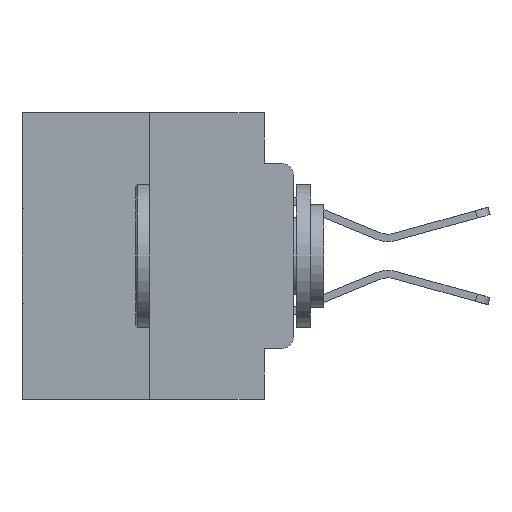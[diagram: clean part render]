
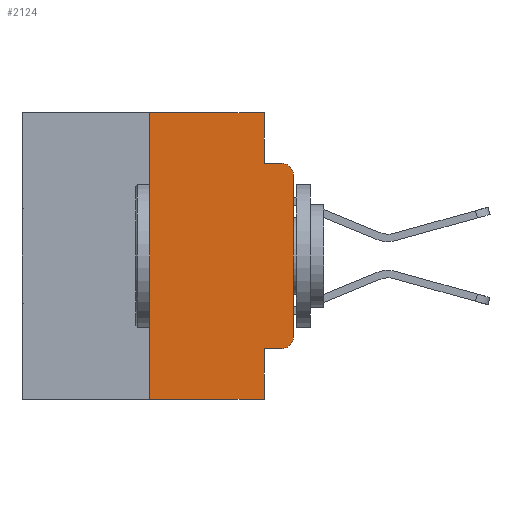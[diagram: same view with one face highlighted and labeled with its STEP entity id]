
A CAD part, left-side view. The second image highlights one B-rep face of the part: STEP entity #2124.
In plain terms, the highlighted planar face has unit normal (-1, 0, 0).
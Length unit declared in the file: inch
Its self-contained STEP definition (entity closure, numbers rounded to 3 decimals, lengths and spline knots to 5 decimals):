
#1100 = CARTESIAN_POINT ( 'NONE',  ( 0., 0.02, -0.4115 ) ) ;
#1102 = CARTESIAN_POINT ( 'NONE',  ( 0., 0., -0.3915 ) ) ;
#1301 = VERTEX_POINT ( 'NONE', #28978 ) ;
#1365 = DIRECTION ( 'NONE',  ( 0., 0., -1. ) ) ;
#1378 = EDGE_CURVE ( 'NONE', #5796, #15668, #2457, .T. ) ;
#1748 = CARTESIAN_POINT ( 'NONE',  ( 0., 0.25, 0. ) ) ;
#1887 = CARTESIAN_POINT ( 'NONE',  ( 0., 0.051, -0.0885 ) ) ;
#1997 = DIRECTION ( 'NONE',  ( -1., 0., 0. ) ) ;
#2112 = ORIENTED_EDGE ( 'NONE', *, *, #6102, .T. ) ;
#2124 = ADVANCED_FACE ( 'NONE', ( #12928 ), #16229, .F. ) ;
#2457 = LINE ( 'NONE', #1887, #20189 ) ;
#2640 = DIRECTION ( 'NONE',  ( 0., -1., 0. ) ) ;
#2888 = CARTESIAN_POINT ( 'NONE',  ( 0., 0.051, -0.0885 ) ) ;
#3114 = LINE ( 'NONE', #1748, #26795 ) ;
#3273 = VECTOR ( 'NONE', #23476, 39.37008 ) ;
#3896 = CARTESIAN_POINT ( 'NONE',  ( 0., 0.051, -0.4115 ) ) ;
#4103 = VECTOR ( 'NONE', #1365, 39.37008 ) ;
#4521 = EDGE_CURVE ( 'NONE', #17932, #15668, #16474, .T. ) ;
#4847 = LINE ( 'NONE', #28804, #4103 ) ;
#5796 = VERTEX_POINT ( 'NONE', #2888 ) ;
#6102 = EDGE_CURVE ( 'NONE', #15426, #17932, #23498, .T. ) ;
#6878 = ORIENTED_EDGE ( 'NONE', *, *, #26819, .T. ) ;
#6981 = VECTOR ( 'NONE', #29676, 39.37008 ) ;
#7036 = CARTESIAN_POINT ( 'NONE',  ( 0., 0.473, 0. ) ) ;
#7969 = AXIS2_PLACEMENT_3D ( 'NONE', #15907, #1997, #18211 ) ;
#8271 = EDGE_CURVE ( 'NONE', #11096, #24901, #26843, .T. ) ;
#9489 = CARTESIAN_POINT ( 'NONE',  ( 0., 0.473, 0. ) ) ;
#9795 = EDGE_CURVE ( 'NONE', #24345, #18157, #3114, .T. ) ;
#10985 = DIRECTION ( 'NONE',  ( 0., -1., 0. ) ) ;
#11096 = VERTEX_POINT ( 'NONE', #3896 ) ;
#11794 = DIRECTION ( 'NONE',  ( 0., 0., -1. ) ) ;
#12287 = ORIENTED_EDGE ( 'NONE', *, *, #28628, .T. ) ;
#12374 = CARTESIAN_POINT ( 'NONE',  ( 0., 0.25, 0. ) ) ;
#12656 = DIRECTION ( 'NONE',  ( -1., 0., 0. ) ) ;
#12928 = FACE_OUTER_BOUND ( 'NONE', #15878, .T. ) ;
#15426 = VERTEX_POINT ( 'NONE', #1102 ) ;
#15502 = ORIENTED_EDGE ( 'NONE', *, *, #4521, .T. ) ;
#15606 = LINE ( 'NONE', #21165, #3273 ) ;
#15668 = VERTEX_POINT ( 'NONE', #24883 ) ;
#15878 = EDGE_LOOP ( 'NONE', ( #2112, #15502, #27550, #16225, #17681, #23745, #6878, #25146, #12287, #24470 ) ) ;
#15907 = CARTESIAN_POINT ( 'NONE',  ( 0., 0.02, -0.1085 ) ) ;
#15942 = DIRECTION ( 'NONE',  ( 0., 0., 1. ) ) ;
#16225 = ORIENTED_EDGE ( 'NONE', *, *, #20576, .F. ) ;
#16229 = PLANE ( 'NONE',  #29215 ) ;
#16474 = CIRCLE ( 'NONE', #7969, 0.02 ) ;
#16707 = VECTOR ( 'NONE', #15942, 39.37008 ) ;
#16919 = AXIS2_PLACEMENT_3D ( 'NONE', #26324, #12656, #28537 ) ;
#17176 = LINE ( 'NONE', #22412, #22518 ) ;
#17681 = ORIENTED_EDGE ( 'NONE', *, *, #28505, .F. ) ;
#17932 = VERTEX_POINT ( 'NONE', #22919 ) ;
#18157 = VERTEX_POINT ( 'NONE', #12374 ) ;
#18211 = DIRECTION ( 'NONE',  ( 0., 0., -1. ) ) ;
#18951 = CARTESIAN_POINT ( 'NONE',  ( 0., 0.051, 0. ) ) ;
#19216 = LINE ( 'NONE', #7036, #6981 ) ;
#19534 = CARTESIAN_POINT ( 'NONE',  ( 0., 0.25, -0.5 ) ) ;
#19863 = VERTEX_POINT ( 'NONE', #1100 ) ;
#20155 = VECTOR ( 'NONE', #25693, 39.37008 ) ;
#20189 = VECTOR ( 'NONE', #2640, 39.37008 ) ;
#20576 = EDGE_CURVE ( 'NONE', #1301, #5796, #4847, .T. ) ;
#21165 = CARTESIAN_POINT ( 'NONE',  ( 0., 0.051, -0.4115 ) ) ;
#21589 = CARTESIAN_POINT ( 'NONE',  ( 0., 0.051, -0.5 ) ) ;
#22412 = CARTESIAN_POINT ( 'NONE',  ( 0., 0.473, -0.5 ) ) ;
#22518 = VECTOR ( 'NONE', #10985, 39.37008 ) ;
#22558 = DIRECTION ( 'NONE',  ( 0., 0., 1. ) ) ;
#22919 = CARTESIAN_POINT ( 'NONE',  ( 0., 0., -0.1085 ) ) ;
#23476 = DIRECTION ( 'NONE',  ( 0., -1., 0. ) ) ;
#23498 = LINE ( 'NONE', #29538, #16707 ) ;
#23745 = ORIENTED_EDGE ( 'NONE', *, *, #9795, .F. ) ;
#24345 = VERTEX_POINT ( 'NONE', #19534 ) ;
#24470 = ORIENTED_EDGE ( 'NONE', *, *, #27162, .T. ) ;
#24883 = CARTESIAN_POINT ( 'NONE',  ( 0., 0.02, -0.0885 ) ) ;
#24901 = VERTEX_POINT ( 'NONE', #21589 ) ;
#25146 = ORIENTED_EDGE ( 'NONE', *, *, #8271, .F. ) ;
#25482 = DIRECTION ( 'NONE',  ( 1., 0., 0. ) ) ;
#25693 = DIRECTION ( 'NONE',  ( 0., 0., -1. ) ) ;
#26021 = CIRCLE ( 'NONE', #16919, 0.02 ) ;
#26324 = CARTESIAN_POINT ( 'NONE',  ( 0., 0.02, -0.3915 ) ) ;
#26795 = VECTOR ( 'NONE', #22558, 39.37008 ) ;
#26819 = EDGE_CURVE ( 'NONE', #24345, #24901, #17176, .T. ) ;
#26843 = LINE ( 'NONE', #18951, #20155 ) ;
#27162 = EDGE_CURVE ( 'NONE', #19863, #15426, #26021, .T. ) ;
#27550 = ORIENTED_EDGE ( 'NONE', *, *, #1378, .F. ) ;
#28505 = EDGE_CURVE ( 'NONE', #18157, #1301, #19216, .T. ) ;
#28537 = DIRECTION ( 'NONE',  ( 0., 0., -1. ) ) ;
#28628 = EDGE_CURVE ( 'NONE', #11096, #19863, #15606, .T. ) ;
#28804 = CARTESIAN_POINT ( 'NONE',  ( 0., 0.051, 0. ) ) ;
#28978 = CARTESIAN_POINT ( 'NONE',  ( 0., 0.051, 0. ) ) ;
#29215 = AXIS2_PLACEMENT_3D ( 'NONE', #9489, #25482, #11794 ) ;
#29538 = CARTESIAN_POINT ( 'NONE',  ( 0., 0., 0. ) ) ;
#29676 = DIRECTION ( 'NONE',  ( 0., -1., 0. ) ) ;
